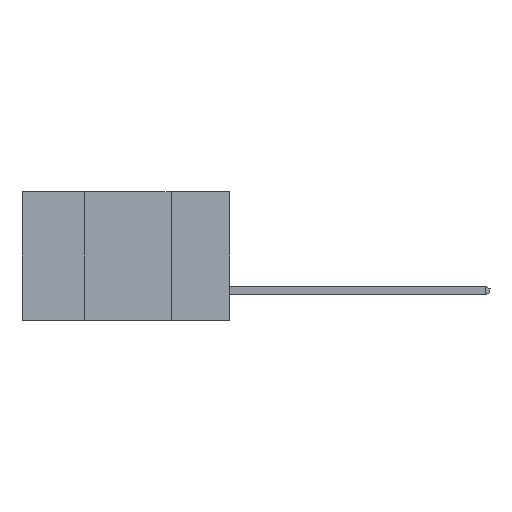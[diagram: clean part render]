
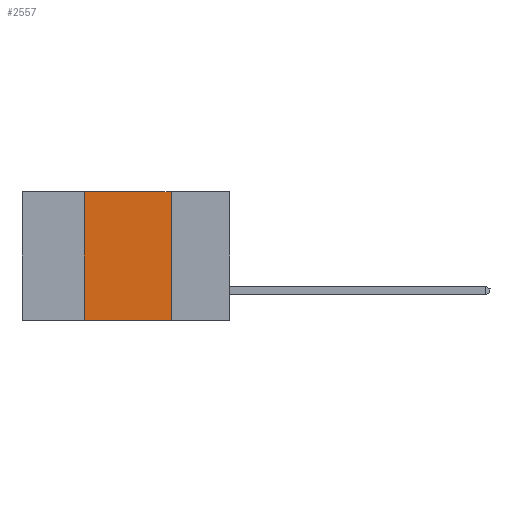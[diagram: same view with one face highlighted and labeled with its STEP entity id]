
A CAD part, left-side view. The second image highlights one B-rep face of the part: STEP entity #2557.
In plain terms, the highlighted planar face has unit normal (-1, 0, 0).
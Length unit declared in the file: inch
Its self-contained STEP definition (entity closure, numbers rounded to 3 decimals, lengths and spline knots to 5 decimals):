
#484 = DIRECTION ( 'NONE',  ( 0., 0., -1. ) ) ;
#890 = ORIENTED_EDGE ( 'NONE', *, *, #3373, .F. ) ;
#894 = EDGE_CURVE ( 'NONE', #9809, #12216, #3277, .T. ) ;
#1227 = VERTEX_POINT ( 'NONE', #12379 ) ;
#1491 = VECTOR ( 'NONE', #7558, 39.37008 ) ;
#2365 = LINE ( 'NONE', #3375, #6909 ) ;
#2424 = CARTESIAN_POINT ( 'NONE',  ( 0., 0.6, 0. ) ) ;
#2433 = DIRECTION ( 'NONE',  ( 0., 0., 1. ) ) ;
#2557 = ADVANCED_FACE ( 'NONE', ( #10402 ), #11458, .F. ) ;
#2796 = LINE ( 'NONE', #8896, #12932 ) ;
#3203 = DIRECTION ( 'NONE',  ( 0., -1., 0. ) ) ;
#3277 = LINE ( 'NONE', #7258, #11655 ) ;
#3373 = EDGE_CURVE ( 'NONE', #9809, #1227, #2365, .T. ) ;
#3375 = CARTESIAN_POINT ( 'NONE',  ( 0., 0.42, -0.37 ) ) ;
#6375 = CARTESIAN_POINT ( 'NONE',  ( 0., 0.17, -0.37 ) ) ;
#6536 = CARTESIAN_POINT ( 'NONE',  ( 0., 0.6, 0. ) ) ;
#6682 = CARTESIAN_POINT ( 'NONE',  ( 0., 0.17, 0. ) ) ;
#6909 = VECTOR ( 'NONE', #2433, 39.37008 ) ;
#7043 = EDGE_CURVE ( 'NONE', #1227, #8901, #8669, .T. ) ;
#7258 = CARTESIAN_POINT ( 'NONE',  ( 0., 0.6, -0.37 ) ) ;
#7276 = CARTESIAN_POINT ( 'NONE',  ( 0., 0.42, -0.37 ) ) ;
#7521 = ORIENTED_EDGE ( 'NONE', *, *, #11834, .F. ) ;
#7558 = DIRECTION ( 'NONE',  ( 0., -1., 0. ) ) ;
#7788 = EDGE_LOOP ( 'NONE', ( #7521, #8002, #890, #11572 ) ) ;
#8002 = ORIENTED_EDGE ( 'NONE', *, *, #7043, .F. ) ;
#8669 = LINE ( 'NONE', #2424, #1491 ) ;
#8896 = CARTESIAN_POINT ( 'NONE',  ( 0., 0.17, -0.37 ) ) ;
#8901 = VERTEX_POINT ( 'NONE', #6682 ) ;
#8966 = DIRECTION ( 'NONE',  ( 0., 0., -1. ) ) ;
#9809 = VERTEX_POINT ( 'NONE', #7276 ) ;
#10402 = FACE_OUTER_BOUND ( 'NONE', #7788, .T. ) ;
#11387 = DIRECTION ( 'NONE',  ( 1., 0., 0. ) ) ;
#11458 = PLANE ( 'NONE',  #12773 ) ;
#11572 = ORIENTED_EDGE ( 'NONE', *, *, #894, .T. ) ;
#11655 = VECTOR ( 'NONE', #3203, 39.37008 ) ;
#11834 = EDGE_CURVE ( 'NONE', #8901, #12216, #2796, .T. ) ;
#12216 = VERTEX_POINT ( 'NONE', #6375 ) ;
#12379 = CARTESIAN_POINT ( 'NONE',  ( 0., 0.42, 0. ) ) ;
#12773 = AXIS2_PLACEMENT_3D ( 'NONE', #6536, #11387, #484 ) ;
#12932 = VECTOR ( 'NONE', #8966, 39.37008 ) ;
